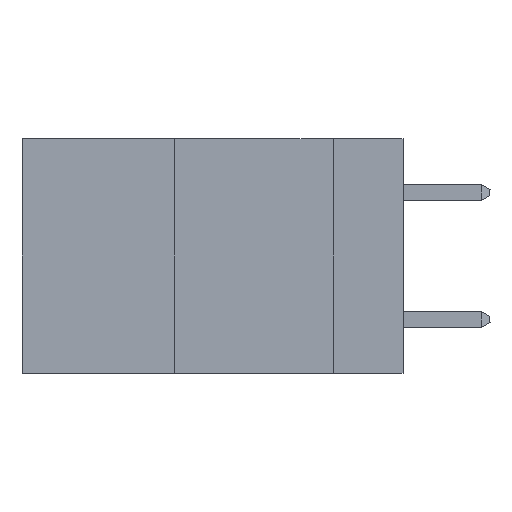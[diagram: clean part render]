
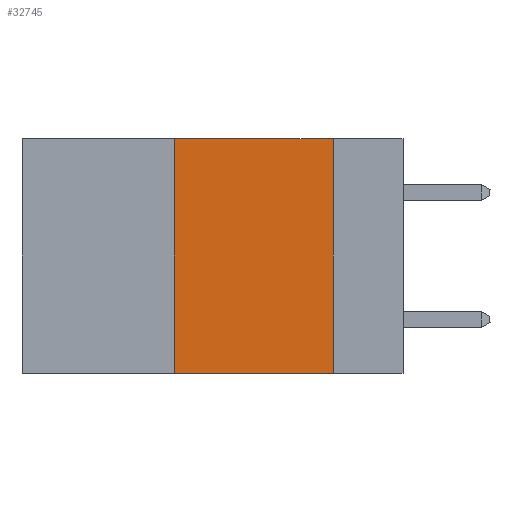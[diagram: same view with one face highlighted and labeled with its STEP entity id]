
A CAD part, left-side view. The second image highlights one B-rep face of the part: STEP entity #32745.
In plain terms, the highlighted planar face has unit normal (-1, 0, 0).
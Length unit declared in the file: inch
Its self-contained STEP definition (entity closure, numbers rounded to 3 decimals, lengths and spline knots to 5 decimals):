
#600 = VERTEX_POINT ( 'NONE', #13680 ) ;
#924 = AXIS2_PLACEMENT_3D ( 'NONE', #33496, #37103, #15555 ) ;
#1046 = CARTESIAN_POINT ( 'NONE',  ( 0., 0.6, -0.37 ) ) ;
#4886 = VERTEX_POINT ( 'NONE', #37632 ) ;
#5439 = CARTESIAN_POINT ( 'NONE',  ( 0., 0.36, 0. ) ) ;
#6033 = VERTEX_POINT ( 'NONE', #40204 ) ;
#7568 = DIRECTION ( 'NONE',  ( 0., 0., -1. ) ) ;
#8286 = PLANE ( 'NONE',  #924 ) ;
#9097 = DIRECTION ( 'NONE',  ( 0., 0., 1. ) ) ;
#10336 = VERTEX_POINT ( 'NONE', #22839 ) ;
#11728 = VECTOR ( 'NONE', #9097, 39.37008 ) ;
#12853 = LINE ( 'NONE', #5439, #11728 ) ;
#13680 = CARTESIAN_POINT ( 'NONE',  ( 0., 0.11, -0.37 ) ) ;
#14799 = EDGE_CURVE ( 'NONE', #4886, #600, #35731, .T. ) ;
#15555 = DIRECTION ( 'NONE',  ( 0., 0., -1. ) ) ;
#16591 = VECTOR ( 'NONE', #26304, 39.37008 ) ;
#18327 = CARTESIAN_POINT ( 'NONE',  ( 0., 0.11, 0. ) ) ;
#22839 = CARTESIAN_POINT ( 'NONE',  ( 0., 0.11, 0. ) ) ;
#26304 = DIRECTION ( 'NONE',  ( 0., -1., 0. ) ) ;
#31847 = VECTOR ( 'NONE', #45853, 39.37008 ) ;
#32745 = ADVANCED_FACE ( 'NONE', ( #35379 ), #8286, .F. ) ;
#33496 = CARTESIAN_POINT ( 'NONE',  ( 0., 0.6, 0. ) ) ;
#33851 = EDGE_CURVE ( 'NONE', #10336, #600, #45408, .T. ) ;
#34616 = EDGE_CURVE ( 'NONE', #6033, #10336, #41396, .T. ) ;
#35379 = FACE_OUTER_BOUND ( 'NONE', #35961, .T. ) ;
#35619 = ORIENTED_EDGE ( 'NONE', *, *, #33851, .F. ) ;
#35731 = LINE ( 'NONE', #1046, #16591 ) ;
#35839 = VECTOR ( 'NONE', #7568, 39.37008 ) ;
#35961 = EDGE_LOOP ( 'NONE', ( #35619, #41838, #36843, #45187 ) ) ;
#36843 = ORIENTED_EDGE ( 'NONE', *, *, #43756, .F. ) ;
#37103 = DIRECTION ( 'NONE',  ( 1., 0., 0. ) ) ;
#37632 = CARTESIAN_POINT ( 'NONE',  ( 0., 0.36, -0.37 ) ) ;
#40204 = CARTESIAN_POINT ( 'NONE',  ( 0., 0.36, 0. ) ) ;
#41396 = LINE ( 'NONE', #42078, #31847 ) ;
#41838 = ORIENTED_EDGE ( 'NONE', *, *, #34616, .F. ) ;
#42078 = CARTESIAN_POINT ( 'NONE',  ( 0., 0.6, 0. ) ) ;
#43756 = EDGE_CURVE ( 'NONE', #4886, #6033, #12853, .T. ) ;
#45187 = ORIENTED_EDGE ( 'NONE', *, *, #14799, .T. ) ;
#45408 = LINE ( 'NONE', #18327, #35839 ) ;
#45853 = DIRECTION ( 'NONE',  ( 0., -1., 0. ) ) ;
